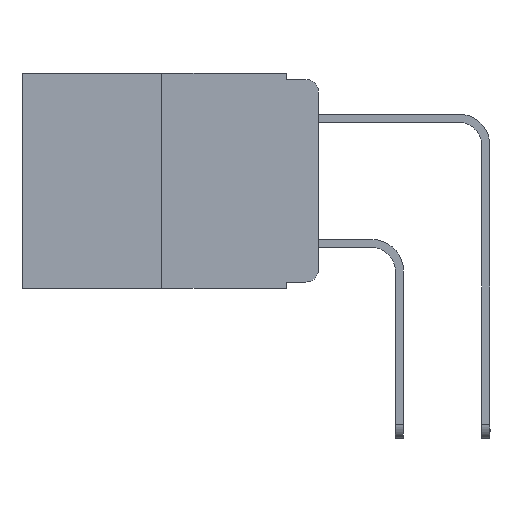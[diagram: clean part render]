
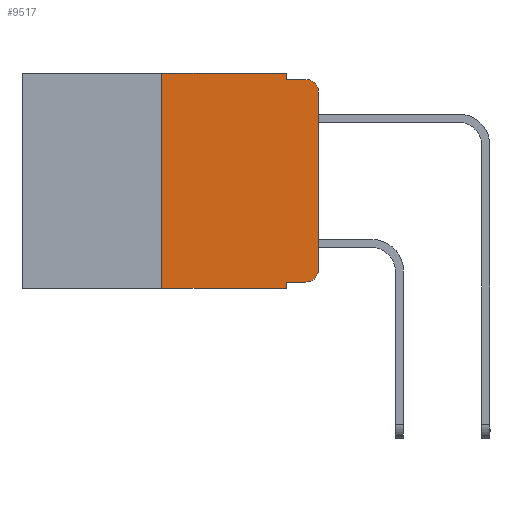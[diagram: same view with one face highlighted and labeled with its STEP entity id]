
A CAD part, left-side view. The second image highlights one B-rep face of the part: STEP entity #9517.
In plain terms, the highlighted planar face has unit normal (-1, 0, 0).
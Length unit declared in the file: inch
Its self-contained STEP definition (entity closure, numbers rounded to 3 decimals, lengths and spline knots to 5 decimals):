
#213 = CARTESIAN_POINT ( 'NONE',  ( 0., 0.051, -0.01 ) ) ;
#301 = LINE ( 'NONE', #3175, #9003 ) ;
#309 = ORIENTED_EDGE ( 'NONE', *, *, #10203, .T. ) ;
#457 = CARTESIAN_POINT ( 'NONE',  ( 0., 0.02, -0.313 ) ) ;
#460 = ORIENTED_EDGE ( 'NONE', *, *, #5435, .F. ) ;
#463 = CARTESIAN_POINT ( 'NONE',  ( 0., 0., 0. ) ) ;
#506 = VECTOR ( 'NONE', #8055, 39.37008 ) ;
#508 = CARTESIAN_POINT ( 'NONE',  ( 0., 0.051, -0.01 ) ) ;
#919 = AXIS2_PLACEMENT_3D ( 'NONE', #3399, #1511, #6321 ) ;
#983 = EDGE_CURVE ( 'NONE', #9725, #4980, #10614, .T. ) ;
#1385 = VERTEX_POINT ( 'NONE', #508 ) ;
#1511 = DIRECTION ( 'NONE',  ( 1., 0., 0. ) ) ;
#1634 = EDGE_CURVE ( 'NONE', #12037, #1385, #5153, .T. ) ;
#1698 = EDGE_CURVE ( 'NONE', #6322, #6665, #8622, .T. ) ;
#1826 = DIRECTION ( 'NONE',  ( 0., 0., -1. ) ) ;
#2127 = LINE ( 'NONE', #6776, #5255 ) ;
#2182 = LINE ( 'NONE', #8327, #12088 ) ;
#2410 = CARTESIAN_POINT ( 'NONE',  ( 0., 0.02, -0.333 ) ) ;
#2623 = EDGE_CURVE ( 'NONE', #6665, #9725, #6886, .T. ) ;
#2861 = DIRECTION ( 'NONE',  ( 0., 0., -1. ) ) ;
#2916 = DIRECTION ( 'NONE',  ( 0., -1., 0. ) ) ;
#3129 = EDGE_CURVE ( 'NONE', #6427, #8263, #301, .T. ) ;
#3139 = ORIENTED_EDGE ( 'NONE', *, *, #2623, .T. ) ;
#3175 = CARTESIAN_POINT ( 'NONE',  ( 0., 0.25, 0. ) ) ;
#3198 = LINE ( 'NONE', #213, #506 ) ;
#3224 = VECTOR ( 'NONE', #5012, 39.37008 ) ;
#3354 = ORIENTED_EDGE ( 'NONE', *, *, #1698, .T. ) ;
#3399 = CARTESIAN_POINT ( 'NONE',  ( 0., 0.473, 0. ) ) ;
#3682 = EDGE_LOOP ( 'NONE', ( #3139, #10280, #6405, #6899, #460, #10328, #6883, #9252, #309, #3354 ) ) ;
#3997 = CARTESIAN_POINT ( 'NONE',  ( 0., 0.02, -0.01 ) ) ;
#4132 = DIRECTION ( 'NONE',  ( 0., 0., -1. ) ) ;
#4229 = DIRECTION ( 'NONE',  ( -1., 0., 0. ) ) ;
#4589 = CARTESIAN_POINT ( 'NONE',  ( 0., 0.051, 0. ) ) ;
#4725 = CARTESIAN_POINT ( 'NONE',  ( 0., 0.25, 0. ) ) ;
#4847 = CARTESIAN_POINT ( 'NONE',  ( 0., 0., -0.03 ) ) ;
#4980 = VERTEX_POINT ( 'NONE', #3997 ) ;
#5012 = DIRECTION ( 'NONE',  ( 0., 0., -1. ) ) ;
#5052 = AXIS2_PLACEMENT_3D ( 'NONE', #457, #4229, #4132 ) ;
#5153 = LINE ( 'NONE', #8763, #3224 ) ;
#5255 = VECTOR ( 'NONE', #7855, 39.37008 ) ;
#5435 = EDGE_CURVE ( 'NONE', #8263, #12037, #2127, .T. ) ;
#5480 = CARTESIAN_POINT ( 'NONE',  ( 0., 0.25, -0.343 ) ) ;
#5906 = VECTOR ( 'NONE', #2916, 39.37008 ) ;
#6071 = LINE ( 'NONE', #7623, #9251 ) ;
#6321 = DIRECTION ( 'NONE',  ( 0., 0., -1. ) ) ;
#6322 = VERTEX_POINT ( 'NONE', #2410 ) ;
#6405 = ORIENTED_EDGE ( 'NONE', *, *, #12290, .F. ) ;
#6427 = VERTEX_POINT ( 'NONE', #5480 ) ;
#6665 = VERTEX_POINT ( 'NONE', #8907 ) ;
#6757 = VECTOR ( 'NONE', #7173, 39.37008 ) ;
#6776 = CARTESIAN_POINT ( 'NONE',  ( 0., 0.473, 0. ) ) ;
#6883 = ORIENTED_EDGE ( 'NONE', *, *, #10039, .T. ) ;
#6886 = LINE ( 'NONE', #463, #6757 ) ;
#6899 = ORIENTED_EDGE ( 'NONE', *, *, #1634, .F. ) ;
#7146 = LINE ( 'NONE', #8613, #5906 ) ;
#7173 = DIRECTION ( 'NONE',  ( 0., 0., 1. ) ) ;
#7221 = PLANE ( 'NONE',  #919 ) ;
#7524 = CARTESIAN_POINT ( 'NONE',  ( 0., 0.051, -0.333 ) ) ;
#7555 = DIRECTION ( 'NONE',  ( -1., 0., 0. ) ) ;
#7623 = CARTESIAN_POINT ( 'NONE',  ( 0., 0.051, 0. ) ) ;
#7834 = EDGE_CURVE ( 'NONE', #12180, #8108, #6071, .T. ) ;
#7855 = DIRECTION ( 'NONE',  ( 0., -1., 0. ) ) ;
#8055 = DIRECTION ( 'NONE',  ( 0., -1., 0. ) ) ;
#8108 = VERTEX_POINT ( 'NONE', #8469 ) ;
#8263 = VERTEX_POINT ( 'NONE', #4725 ) ;
#8327 = CARTESIAN_POINT ( 'NONE',  ( 0., 0.473, -0.343 ) ) ;
#8469 = CARTESIAN_POINT ( 'NONE',  ( 0., 0.051, -0.343 ) ) ;
#8613 = CARTESIAN_POINT ( 'NONE',  ( 0., 0.051, -0.333 ) ) ;
#8622 = CIRCLE ( 'NONE', #5052, 0.02 ) ;
#8763 = CARTESIAN_POINT ( 'NONE',  ( 0., 0.051, 0. ) ) ;
#8907 = CARTESIAN_POINT ( 'NONE',  ( 0., 0., -0.313 ) ) ;
#9003 = VECTOR ( 'NONE', #11810, 39.37008 ) ;
#9251 = VECTOR ( 'NONE', #2861, 39.37008 ) ;
#9252 = ORIENTED_EDGE ( 'NONE', *, *, #7834, .F. ) ;
#9291 = DIRECTION ( 'NONE',  ( 0., -1., 0. ) ) ;
#9517 = ADVANCED_FACE ( 'NONE', ( #9697 ), #7221, .F. ) ;
#9697 = FACE_OUTER_BOUND ( 'NONE', #3682, .T. ) ;
#9725 = VERTEX_POINT ( 'NONE', #4847 ) ;
#10039 = EDGE_CURVE ( 'NONE', #6427, #8108, #2182, .T. ) ;
#10203 = EDGE_CURVE ( 'NONE', #12180, #6322, #7146, .T. ) ;
#10280 = ORIENTED_EDGE ( 'NONE', *, *, #983, .T. ) ;
#10328 = ORIENTED_EDGE ( 'NONE', *, *, #3129, .F. ) ;
#10614 = CIRCLE ( 'NONE', #12152, 0.02 ) ;
#11810 = DIRECTION ( 'NONE',  ( 0., 0., 1. ) ) ;
#12037 = VERTEX_POINT ( 'NONE', #4589 ) ;
#12088 = VECTOR ( 'NONE', #9291, 39.37008 ) ;
#12152 = AXIS2_PLACEMENT_3D ( 'NONE', #12299, #7555, #1826 ) ;
#12180 = VERTEX_POINT ( 'NONE', #7524 ) ;
#12290 = EDGE_CURVE ( 'NONE', #1385, #4980, #3198, .T. ) ;
#12299 = CARTESIAN_POINT ( 'NONE',  ( 0., 0.02, -0.03 ) ) ;
